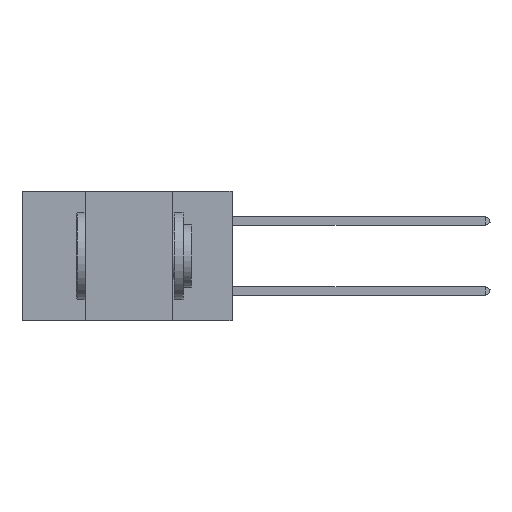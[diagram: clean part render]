
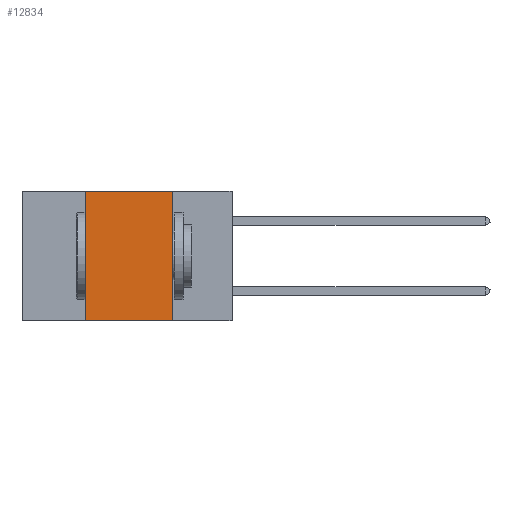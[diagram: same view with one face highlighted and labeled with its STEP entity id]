
A CAD part, left-side view. The second image highlights one B-rep face of the part: STEP entity #12834.
In plain terms, the highlighted planar face has unit normal (-1, 0, 0).
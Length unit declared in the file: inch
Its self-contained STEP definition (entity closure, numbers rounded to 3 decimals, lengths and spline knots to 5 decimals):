
#57 = DIRECTION ( 'NONE',  ( 1., 0., 0. ) ) ;
#760 = CARTESIAN_POINT ( 'NONE',  ( 0., 0.17, -0.37 ) ) ;
#897 = CARTESIAN_POINT ( 'NONE',  ( 0., 0.42, 0. ) ) ;
#941 = EDGE_CURVE ( 'NONE', #10248, #10778, #1206, .T. ) ;
#1206 = LINE ( 'NONE', #6599, #14136 ) ;
#1483 = DIRECTION ( 'NONE',  ( 0., 0., -1. ) ) ;
#2393 = LINE ( 'NONE', #10663, #6267 ) ;
#4096 = CARTESIAN_POINT ( 'NONE',  ( 0., 0.6, -0.37 ) ) ;
#4158 = DIRECTION ( 'NONE',  ( 0., -1., 0. ) ) ;
#4289 = ORIENTED_EDGE ( 'NONE', *, *, #6464, .F. ) ;
#5396 = PLANE ( 'NONE',  #13829 ) ;
#6267 = VECTOR ( 'NONE', #1483, 39.37008 ) ;
#6464 = EDGE_CURVE ( 'NONE', #16629, #10248, #10376, .T. ) ;
#6599 = CARTESIAN_POINT ( 'NONE',  ( 0., 0.6, 0. ) ) ;
#6752 = EDGE_CURVE ( 'NONE', #10778, #11179, #2393, .T. ) ;
#7200 = CARTESIAN_POINT ( 'NONE',  ( 0., 0.42, -0.37 ) ) ;
#8012 = CARTESIAN_POINT ( 'NONE',  ( 0., 0.6, 0. ) ) ;
#8377 = EDGE_CURVE ( 'NONE', #16629, #11179, #12010, .T. ) ;
#8583 = VECTOR ( 'NONE', #4158, 39.37008 ) ;
#8774 = DIRECTION ( 'NONE',  ( 0., 0., 1. ) ) ;
#9298 = DIRECTION ( 'NONE',  ( 0., 0., -1. ) ) ;
#9580 = DIRECTION ( 'NONE',  ( 0., -1., 0. ) ) ;
#10248 = VERTEX_POINT ( 'NONE', #10351 ) ;
#10351 = CARTESIAN_POINT ( 'NONE',  ( 0., 0.42, 0. ) ) ;
#10376 = LINE ( 'NONE', #897, #13324 ) ;
#10663 = CARTESIAN_POINT ( 'NONE',  ( 0., 0.17, 0. ) ) ;
#10778 = VERTEX_POINT ( 'NONE', #11513 ) ;
#11155 = ORIENTED_EDGE ( 'NONE', *, *, #8377, .T. ) ;
#11179 = VERTEX_POINT ( 'NONE', #760 ) ;
#11258 = FACE_OUTER_BOUND ( 'NONE', #12917, .T. ) ;
#11513 = CARTESIAN_POINT ( 'NONE',  ( 0., 0.17, 0. ) ) ;
#12010 = LINE ( 'NONE', #4096, #8583 ) ;
#12834 = ADVANCED_FACE ( 'NONE', ( #11258 ), #5396, .F. ) ;
#12917 = EDGE_LOOP ( 'NONE', ( #13704, #14066, #4289, #11155 ) ) ;
#13324 = VECTOR ( 'NONE', #8774, 39.37008 ) ;
#13704 = ORIENTED_EDGE ( 'NONE', *, *, #6752, .F. ) ;
#13829 = AXIS2_PLACEMENT_3D ( 'NONE', #8012, #57, #9298 ) ;
#14066 = ORIENTED_EDGE ( 'NONE', *, *, #941, .F. ) ;
#14136 = VECTOR ( 'NONE', #9580, 39.37008 ) ;
#16629 = VERTEX_POINT ( 'NONE', #7200 ) ;
